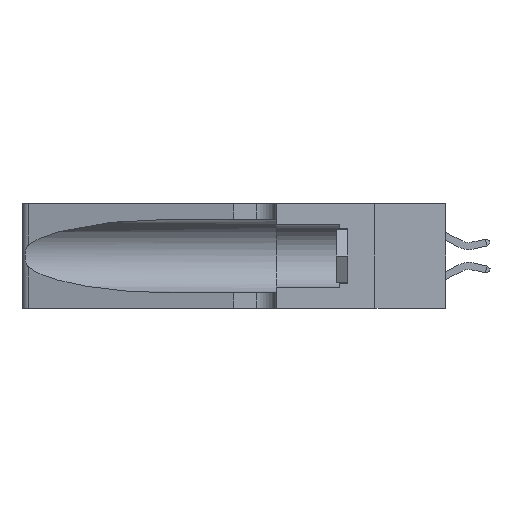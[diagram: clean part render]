
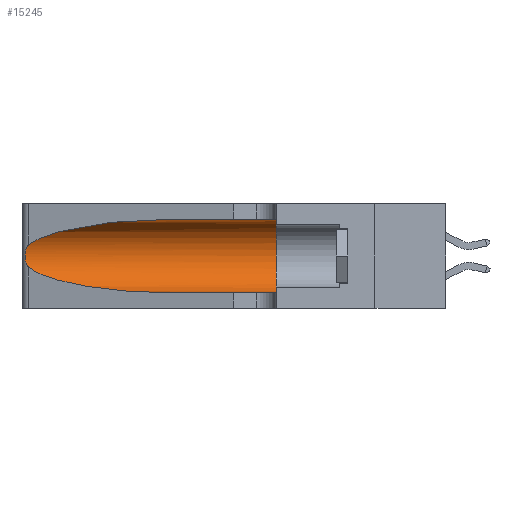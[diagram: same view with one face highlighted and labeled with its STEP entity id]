
A CAD part, left-side view. The second image highlights one B-rep face of the part: STEP entity #15245.
In plain terms, the highlighted cylindrical face has radius 3.308 mm (diameter 6.617 mm), a partial arc.
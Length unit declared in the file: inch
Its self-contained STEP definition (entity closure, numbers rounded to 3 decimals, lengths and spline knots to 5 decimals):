
#226 = CARTESIAN_POINT ( 'NONE',  ( 0.25487, 1.22718, 0.22369 ) ) ;
#431 = DIRECTION ( 'NONE',  ( 0., -1., 0. ) ) ;
#458 = DIRECTION ( 'NONE',  ( 0., 1., 0. ) ) ;
#549 = VERTEX_POINT ( 'NONE', #20723 ) ;
#927 = CARTESIAN_POINT ( 'NONE',  ( 0.26018, 1.23835, 0.19895 ) ) ;
#1965 = DIRECTION ( 'NONE',  ( 0., -1., 0. ) ) ;
#2024 = ORIENTED_EDGE ( 'NONE', *, *, #24922, .T. ) ;
#2312 = EDGE_CURVE ( 'NONE', #15179, #17309, #9902, .T. ) ;
#2326 = CARTESIAN_POINT ( 'NONE',  ( 0.25555, 1.22994, 0.2215 ) ) ;
#2574 = DIRECTION ( 'NONE',  ( 0., 0., 1. ) ) ;
#2623 = CARTESIAN_POINT ( 'NONE',  ( 0.25487, 1.22718, 0.14631 ) ) ;
#3124 = CARTESIAN_POINT ( 'NONE',  ( 0.18966, 0.96281, 0.31525 ) ) ;
#3202 = CARTESIAN_POINT ( 'NONE',  ( 0.25487, 1.22718, 0.22369 ) ) ;
#3735 = CARTESIAN_POINT ( 'NONE',  ( 0.25487, 1.22718, 0.22369 ) ) ;
#3935 = CARTESIAN_POINT ( 'NONE',  ( 0.25487, 1.22718, 0.14631 ) ) ;
#4156 = AXIS2_PLACEMENT_3D ( 'NONE', #14851, #10634, #25159 ) ;
#5065 =( BOUNDED_CURVE ( )  B_SPLINE_CURVE ( 3, ( #12066, #7603, #22107, #15889 ),
 .UNSPECIFIED., .F., .F. ) 
 B_SPLINE_CURVE_WITH_KNOTS ( ( 4, 4 ),
 ( 3.44316, 4.71239 ),
 .UNSPECIFIED. ) 
 CURVE ( )  GEOMETRIC_REPRESENTATION_ITEM ( )  RATIONAL_B_SPLINE_CURVE ( ( 1., 0.87, 0.87, 1. ) ) 
 REPRESENTATION_ITEM ( '' )  );
#5203 = CARTESIAN_POINT ( 'NONE',  ( 0.26075, 1.23896, 0.19203 ) ) ;
#5311 = CYLINDRICAL_SURFACE ( 'NONE', #4156, 0.13025 ) ;
#5440 = ORIENTED_EDGE ( 'NONE', *, *, #10753, .T. ) ;
#5550 = B_SPLINE_CURVE_WITH_KNOTS ( 'NONE', 3,
 ( #3735, #2326, #16847, #21527, #25819, #927, #5203, #19932, #17664, #21906, #13731, #24539, #26696, #3935 ),
 .UNSPECIFIED., .F., .F.,
 ( 4, 2, 2, 2, 2, 2, 4 ),
 ( 0., 0.00027, 0.00053, 0.00107, 0.0016, 0.00187, 0.00214 ),
 .UNSPECIFIED. ) ;
#5614 = ORIENTED_EDGE ( 'NONE', *, *, #2312, .T. ) ;
#6239 = CARTESIAN_POINT ( 'NONE',  ( 0.1305, 0.35, 0.31525 ) ) ;
#6361 = CARTESIAN_POINT ( 'NONE',  ( 0.1305, 0.72297, 0.31525 ) ) ;
#6717 = ORIENTED_EDGE ( 'NONE', *, *, #7376, .T. ) ;
#7376 = EDGE_CURVE ( 'NONE', #17309, #22117, #5550, .T. ) ;
#7603 = CARTESIAN_POINT ( 'NONE',  ( 0.2373, 1.15595, 0.08982 ) ) ;
#7776 = ORIENTED_EDGE ( 'NONE', *, *, #26847, .F. ) ;
#8596 = EDGE_LOOP ( 'NONE', ( #5614, #6717, #5440, #2024, #13923, #7776 ) ) ;
#9902 =( BOUNDED_CURVE ( )  B_SPLINE_CURVE ( 3, ( #13626, #3124, #25973, #3202 ),
 .UNSPECIFIED., .F., .T. ) 
 B_SPLINE_CURVE_WITH_KNOTS ( ( 4, 4 ),
 ( 1.5708, 2.84003 ),
 .UNSPECIFIED. ) 
 CURVE ( )  GEOMETRIC_REPRESENTATION_ITEM ( )  RATIONAL_B_SPLINE_CURVE ( ( 1., 0.87, 0.87, 1. ) ) 
 REPRESENTATION_ITEM ( '' )  );
#10634 = DIRECTION ( 'NONE',  ( 0., -1., 0. ) ) ;
#10753 = EDGE_CURVE ( 'NONE', #22117, #20465, #5065, .T. ) ;
#12066 = CARTESIAN_POINT ( 'NONE',  ( 0.25487, 1.22718, 0.14631 ) ) ;
#12327 = CARTESIAN_POINT ( 'NONE',  ( 0.1305, 1.61858, 0.05475 ) ) ;
#12921 = CARTESIAN_POINT ( 'NONE',  ( 0.1305, 0.35, 0.185 ) ) ;
#13090 = EDGE_CURVE ( 'NONE', #22509, #549, #26862, .T. ) ;
#13626 = CARTESIAN_POINT ( 'NONE',  ( 0.1305, 0.72297, 0.31525 ) ) ;
#13731 = CARTESIAN_POINT ( 'NONE',  ( 0.25789, 1.23486, 0.15765 ) ) ;
#13793 = CARTESIAN_POINT ( 'NONE',  ( 0.1305, 0.72297, 0.05475 ) ) ;
#13923 = ORIENTED_EDGE ( 'NONE', *, *, #13090, .F. ) ;
#14851 = CARTESIAN_POINT ( 'NONE',  ( 0.1305, 1.61858, 0.185 ) ) ;
#15179 = VERTEX_POINT ( 'NONE', #6361 ) ;
#15245 = ADVANCED_FACE ( 'NONE', ( #18872 ), #5311, .F. ) ;
#15562 = CARTESIAN_POINT ( 'NONE',  ( 0.1305, 1.61858, 0.31525 ) ) ;
#15715 = VECTOR ( 'NONE', #1965, 39.37008 ) ;
#15889 = CARTESIAN_POINT ( 'NONE',  ( 0.1305, 0.72297, 0.05475 ) ) ;
#16847 = CARTESIAN_POINT ( 'NONE',  ( 0.25639, 1.23184, 0.21858 ) ) ;
#17309 = VERTEX_POINT ( 'NONE', #226 ) ;
#17664 = CARTESIAN_POINT ( 'NONE',  ( 0.26017, 1.23833, 0.17102 ) ) ;
#18817 = AXIS2_PLACEMENT_3D ( 'NONE', #12921, #458, #2574 ) ;
#18872 = FACE_OUTER_BOUND ( 'NONE', #8596, .T. ) ;
#19932 = CARTESIAN_POINT ( 'NONE',  ( 0.26075, 1.23896, 0.178 ) ) ;
#20465 = VERTEX_POINT ( 'NONE', #13793 ) ;
#20723 = CARTESIAN_POINT ( 'NONE',  ( 0.1305, 0.35, 0.05475 ) ) ;
#20981 = LINE ( 'NONE', #12327, #15715 ) ;
#21527 = CARTESIAN_POINT ( 'NONE',  ( 0.25787, 1.23484, 0.2124 ) ) ;
#21906 = CARTESIAN_POINT ( 'NONE',  ( 0.25856, 1.23593, 0.16098 ) ) ;
#22107 = CARTESIAN_POINT ( 'NONE',  ( 0.18966, 0.96281, 0.05475 ) ) ;
#22117 = VERTEX_POINT ( 'NONE', #2623 ) ;
#22509 = VERTEX_POINT ( 'NONE', #6239 ) ;
#23487 = LINE ( 'NONE', #15562, #26432 ) ;
#24539 = CARTESIAN_POINT ( 'NONE',  ( 0.25639, 1.23186, 0.15144 ) ) ;
#24922 = EDGE_CURVE ( 'NONE', #20465, #549, #20981, .T. ) ;
#25159 = DIRECTION ( 'NONE',  ( 0., 0., -1. ) ) ;
#25819 = CARTESIAN_POINT ( 'NONE',  ( 0.25854, 1.2359, 0.20912 ) ) ;
#25973 = CARTESIAN_POINT ( 'NONE',  ( 0.2373, 1.15595, 0.28018 ) ) ;
#26432 = VECTOR ( 'NONE', #431, 39.37008 ) ;
#26696 = CARTESIAN_POINT ( 'NONE',  ( 0.25555, 1.22993, 0.14849 ) ) ;
#26847 = EDGE_CURVE ( 'NONE', #15179, #22509, #23487, .T. ) ;
#26862 = CIRCLE ( 'NONE', #18817, 0.13025 ) ;
